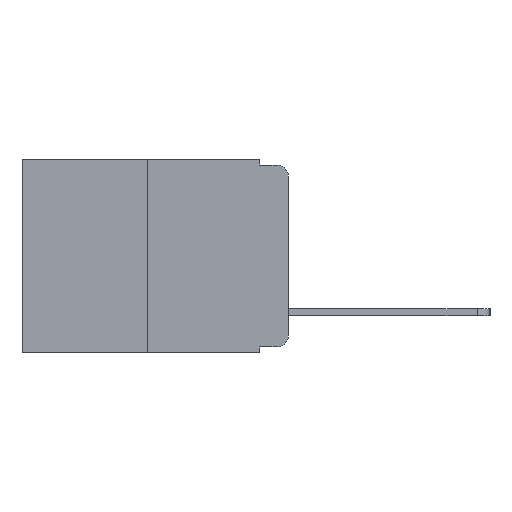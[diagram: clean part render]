
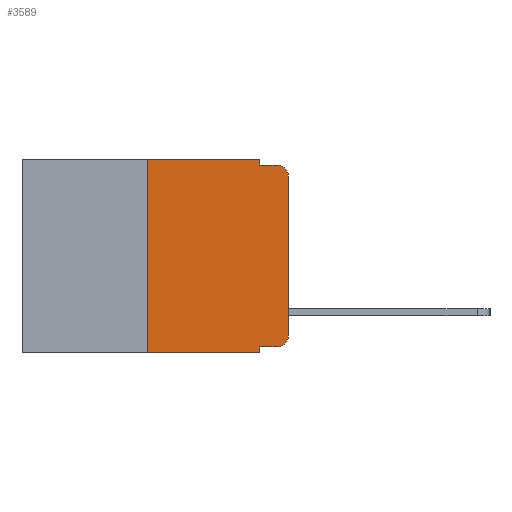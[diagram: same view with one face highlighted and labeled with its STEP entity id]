
A CAD part, left-side view. The second image highlights one B-rep face of the part: STEP entity #3589.
In plain terms, the highlighted planar face has unit normal (-1, 0, 0).
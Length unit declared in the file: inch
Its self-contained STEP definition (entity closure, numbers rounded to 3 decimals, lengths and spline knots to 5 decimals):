
#240 = CARTESIAN_POINT ( 'NONE',  ( 0., 0.051, -0.01 ) ) ;
#390 = CARTESIAN_POINT ( 'NONE',  ( 0., 0.02, -0.03 ) ) ;
#770 = CARTESIAN_POINT ( 'NONE',  ( 0., 0., -0.313 ) ) ;
#812 = VECTOR ( 'NONE', #16294, 39.37008 ) ;
#1554 = DIRECTION ( 'NONE',  ( 0., -1., 0. ) ) ;
#1761 = EDGE_LOOP ( 'NONE', ( #20552, #21762, #14450, #20865, #13543, #9601, #12626, #4129, #21503, #7198 ) ) ;
#2009 = CARTESIAN_POINT ( 'NONE',  ( 0., 0.25, -0.343 ) ) ;
#2112 = VERTEX_POINT ( 'NONE', #21658 ) ;
#2343 = DIRECTION ( 'NONE',  ( 0., 0., -1. ) ) ;
#2829 = EDGE_CURVE ( 'NONE', #9497, #16679, #25148, .T. ) ;
#3291 = DIRECTION ( 'NONE',  ( 0., 0., -1. ) ) ;
#3483 = VECTOR ( 'NONE', #5989, 39.37008 ) ;
#3589 = ADVANCED_FACE ( 'NONE', ( #16308 ), #6967, .F. ) ;
#3850 = CARTESIAN_POINT ( 'NONE',  ( 0., 0.02, -0.333 ) ) ;
#4129 = ORIENTED_EDGE ( 'NONE', *, *, #6263, .F. ) ;
#4191 = CARTESIAN_POINT ( 'NONE',  ( 0., 0., 0. ) ) ;
#5987 = AXIS2_PLACEMENT_3D ( 'NONE', #390, #14029, #2343 ) ;
#5989 = DIRECTION ( 'NONE',  ( 0., -1., 0. ) ) ;
#6035 = LINE ( 'NONE', #24032, #812 ) ;
#6263 = EDGE_CURVE ( 'NONE', #9497, #9850, #20160, .T. ) ;
#6452 = LINE ( 'NONE', #12519, #21371 ) ;
#6645 = CARTESIAN_POINT ( 'NONE',  ( 0., 0.051, -0.333 ) ) ;
#6761 = DIRECTION ( 'NONE',  ( 0., 0., 1. ) ) ;
#6967 = PLANE ( 'NONE',  #16129 ) ;
#7198 = ORIENTED_EDGE ( 'NONE', *, *, #19409, .T. ) ;
#8011 = VERTEX_POINT ( 'NONE', #9554 ) ;
#9497 = VERTEX_POINT ( 'NONE', #16426 ) ;
#9554 = CARTESIAN_POINT ( 'NONE',  ( 0., 0.02, -0.01 ) ) ;
#9601 = ORIENTED_EDGE ( 'NONE', *, *, #11247, .F. ) ;
#9693 = CIRCLE ( 'NONE', #5987, 0.02 ) ;
#9706 = VECTOR ( 'NONE', #20262, 39.37008 ) ;
#9828 = CARTESIAN_POINT ( 'NONE',  ( 0., 0.25, 0. ) ) ;
#9850 = VERTEX_POINT ( 'NONE', #11750 ) ;
#10363 = CARTESIAN_POINT ( 'NONE',  ( 0., 0.02, -0.313 ) ) ;
#10688 = VERTEX_POINT ( 'NONE', #16186 ) ;
#11091 = EDGE_CURVE ( 'NONE', #2112, #21106, #15256, .T. ) ;
#11247 = EDGE_CURVE ( 'NONE', #17347, #13394, #6452, .T. ) ;
#11444 = CARTESIAN_POINT ( 'NONE',  ( 0., 0.473, -0.343 ) ) ;
#11750 = CARTESIAN_POINT ( 'NONE',  ( 0., 0.051, -0.343 ) ) ;
#12302 = DIRECTION ( 'NONE',  ( 0., 0., -1. ) ) ;
#12519 = CARTESIAN_POINT ( 'NONE',  ( 0., 0.25, 0. ) ) ;
#12626 = ORIENTED_EDGE ( 'NONE', *, *, #23264, .T. ) ;
#12802 = DIRECTION ( 'NONE',  ( 0., 0., -1. ) ) ;
#12984 = CARTESIAN_POINT ( 'NONE',  ( 0., 0.051, 0. ) ) ;
#13129 = CIRCLE ( 'NONE', #24920, 0.02 ) ;
#13394 = VERTEX_POINT ( 'NONE', #9828 ) ;
#13543 = ORIENTED_EDGE ( 'NONE', *, *, #14249, .F. ) ;
#14029 = DIRECTION ( 'NONE',  ( -1., 0., 0. ) ) ;
#14141 = EDGE_CURVE ( 'NONE', #10688, #8011, #9693, .T. ) ;
#14249 = EDGE_CURVE ( 'NONE', #13394, #2112, #6035, .T. ) ;
#14362 = VECTOR ( 'NONE', #3291, 39.37008 ) ;
#14450 = ORIENTED_EDGE ( 'NONE', *, *, #16795, .F. ) ;
#14498 = VECTOR ( 'NONE', #1554, 39.37008 ) ;
#14666 = VECTOR ( 'NONE', #17442, 39.37008 ) ;
#15088 = LINE ( 'NONE', #11444, #14498 ) ;
#15256 = LINE ( 'NONE', #23337, #14666 ) ;
#16129 = AXIS2_PLACEMENT_3D ( 'NONE', #16612, #24408, #12802 ) ;
#16186 = CARTESIAN_POINT ( 'NONE',  ( 0., 0., -0.03 ) ) ;
#16294 = DIRECTION ( 'NONE',  ( 0., -1., 0. ) ) ;
#16308 = FACE_OUTER_BOUND ( 'NONE', #1761, .T. ) ;
#16426 = CARTESIAN_POINT ( 'NONE',  ( 0., 0.051, -0.333 ) ) ;
#16612 = CARTESIAN_POINT ( 'NONE',  ( 0., 0.473, 0. ) ) ;
#16679 = VERTEX_POINT ( 'NONE', #3850 ) ;
#16795 = EDGE_CURVE ( 'NONE', #21106, #8011, #24154, .T. ) ;
#17347 = VERTEX_POINT ( 'NONE', #2009 ) ;
#17442 = DIRECTION ( 'NONE',  ( 0., 0., -1. ) ) ;
#18798 = LINE ( 'NONE', #4191, #23371 ) ;
#19409 = EDGE_CURVE ( 'NONE', #16679, #20164, #13129, .T. ) ;
#20160 = LINE ( 'NONE', #12984, #14362 ) ;
#20164 = VERTEX_POINT ( 'NONE', #770 ) ;
#20262 = DIRECTION ( 'NONE',  ( 0., -1., 0. ) ) ;
#20552 = ORIENTED_EDGE ( 'NONE', *, *, #22211, .T. ) ;
#20865 = ORIENTED_EDGE ( 'NONE', *, *, #11091, .F. ) ;
#21106 = VERTEX_POINT ( 'NONE', #21193 ) ;
#21193 = CARTESIAN_POINT ( 'NONE',  ( 0., 0.051, -0.01 ) ) ;
#21371 = VECTOR ( 'NONE', #6761, 39.37008 ) ;
#21503 = ORIENTED_EDGE ( 'NONE', *, *, #2829, .T. ) ;
#21649 = DIRECTION ( 'NONE',  ( 0., 0., 1. ) ) ;
#21658 = CARTESIAN_POINT ( 'NONE',  ( 0., 0.051, 0. ) ) ;
#21762 = ORIENTED_EDGE ( 'NONE', *, *, #14141, .T. ) ;
#22211 = EDGE_CURVE ( 'NONE', #20164, #10688, #18798, .T. ) ;
#23264 = EDGE_CURVE ( 'NONE', #17347, #9850, #15088, .T. ) ;
#23337 = CARTESIAN_POINT ( 'NONE',  ( 0., 0.051, 0. ) ) ;
#23371 = VECTOR ( 'NONE', #21649, 39.37008 ) ;
#23945 = DIRECTION ( 'NONE',  ( -1., 0., 0. ) ) ;
#24032 = CARTESIAN_POINT ( 'NONE',  ( 0., 0.473, 0. ) ) ;
#24154 = LINE ( 'NONE', #240, #3483 ) ;
#24408 = DIRECTION ( 'NONE',  ( 1., 0., 0. ) ) ;
#24920 = AXIS2_PLACEMENT_3D ( 'NONE', #10363, #23945, #12302 ) ;
#25148 = LINE ( 'NONE', #6645, #9706 ) ;
